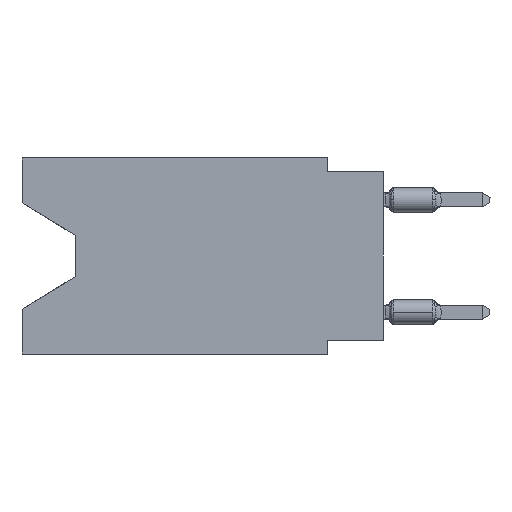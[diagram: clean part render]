
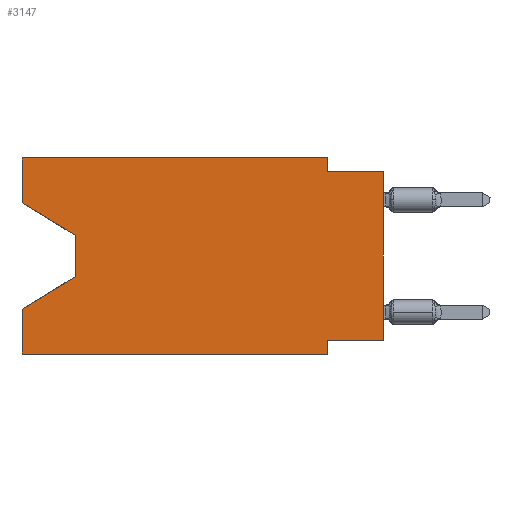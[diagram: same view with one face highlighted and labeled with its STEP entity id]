
A CAD part, left-side view. The second image highlights one B-rep face of the part: STEP entity #3147.
In plain terms, the highlighted planar face has unit normal (-1, 0, 0).
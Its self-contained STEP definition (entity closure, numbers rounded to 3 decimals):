
#388 = EDGE_CURVE ( 'NONE', #33788, #4789, #6880, .T. ) ;
#556 = LINE ( 'NONE', #11380, #32967 ) ;
#1102 = VERTEX_POINT ( 'NONE', #30355 ) ;
#1315 = CARTESIAN_POINT ( 'NONE',  ( 0., 16.383, -8.89 ) ) ;
#1552 = CARTESIAN_POINT ( 'NONE',  ( 0., 16.383, 0. ) ) ;
#1787 = CARTESIAN_POINT ( 'NONE',  ( 0., 0., -8.255 ) ) ;
#2194 = CARTESIAN_POINT ( 'NONE',  ( 0., 16.383, -6.852 ) ) ;
#2644 = VERTEX_POINT ( 'NONE', #27461 ) ;
#3091 = LINE ( 'NONE', #11064, #3766 ) ;
#3147 = ADVANCED_FACE ( 'NONE', ( #27585 ), #18928, .F. ) ;
#3168 = EDGE_CURVE ( 'NONE', #2644, #5817, #12613, .T. ) ;
#3664 = DIRECTION ( 'NONE',  ( 0., 0., -1. ) ) ;
#3766 = VECTOR ( 'NONE', #27421, 1000. ) ;
#4789 = VERTEX_POINT ( 'NONE', #25875 ) ;
#4899 = DIRECTION ( 'NONE',  ( 0., 0., 1. ) ) ;
#5340 = ORIENTED_EDGE ( 'NONE', *, *, #31340, .F. ) ;
#5543 = EDGE_CURVE ( 'NONE', #34579, #11997, #10096, .T. ) ;
#5817 = VERTEX_POINT ( 'NONE', #25352 ) ;
#6232 = VECTOR ( 'NONE', #12568, 1000. ) ;
#6847 = CARTESIAN_POINT ( 'NONE',  ( 0., 13.97, -3.505 ) ) ;
#6880 = LINE ( 'NONE', #1552, #6232 ) ;
#7727 = LINE ( 'NONE', #29780, #26782 ) ;
#8741 = DIRECTION ( 'NONE',  ( 0., 1., 0. ) ) ;
#8787 = CARTESIAN_POINT ( 'NONE',  ( 0., 16.383, 0. ) ) ;
#9070 = VERTEX_POINT ( 'NONE', #15032 ) ;
#9883 = DIRECTION ( 'NONE',  ( 0., -0.855, -0.519 ) ) ;
#10096 = LINE ( 'NONE', #15995, #27792 ) ;
#10443 = EDGE_CURVE ( 'NONE', #27544, #33788, #29067, .T. ) ;
#10603 = ORIENTED_EDGE ( 'NONE', *, *, #388, .F. ) ;
#10645 = CARTESIAN_POINT ( 'NONE',  ( 0., 2.54, -8.89 ) ) ;
#10707 = ORIENTED_EDGE ( 'NONE', *, *, #33769, .T. ) ;
#11064 = CARTESIAN_POINT ( 'NONE',  ( 0., 2.54, 0. ) ) ;
#11380 = CARTESIAN_POINT ( 'NONE',  ( 0., 0., -0.635 ) ) ;
#11549 = DIRECTION ( 'NONE',  ( 0., -1., 0. ) ) ;
#11997 = VERTEX_POINT ( 'NONE', #2194 ) ;
#12079 = AXIS2_PLACEMENT_3D ( 'NONE', #32952, #13908, #21577 ) ;
#12568 = DIRECTION ( 'NONE',  ( 0., -1., 0. ) ) ;
#12613 = LINE ( 'NONE', #1787, #19463 ) ;
#13866 = ORIENTED_EDGE ( 'NONE', *, *, #27496, .T. ) ;
#13908 = DIRECTION ( 'NONE',  ( 1., 0., 0. ) ) ;
#14046 = VECTOR ( 'NONE', #3664, 1000. ) ;
#14711 = ORIENTED_EDGE ( 'NONE', *, *, #5543, .F. ) ;
#15032 = CARTESIAN_POINT ( 'NONE',  ( 0., 2.54, -0.635 ) ) ;
#15124 = CARTESIAN_POINT ( 'NONE',  ( 0., 2.54, -8.89 ) ) ;
#15523 = ORIENTED_EDGE ( 'NONE', *, *, #22405, .T. ) ;
#15639 = LINE ( 'NONE', #10645, #22576 ) ;
#15821 = DIRECTION ( 'NONE',  ( 0., 0., -1. ) ) ;
#15981 = CARTESIAN_POINT ( 'NONE',  ( 0., 13.97, -5.385 ) ) ;
#15995 = CARTESIAN_POINT ( 'NONE',  ( 0., 16.383, 0. ) ) ;
#16669 = LINE ( 'NONE', #15981, #30411 ) ;
#17548 = LINE ( 'NONE', #26055, #21049 ) ;
#18928 = PLANE ( 'NONE',  #12079 ) ;
#19033 = EDGE_CURVE ( 'NONE', #24643, #11997, #16669, .T. ) ;
#19463 = VECTOR ( 'NONE', #8741, 1000. ) ;
#20163 = VECTOR ( 'NONE', #4899, 1000. ) ;
#20191 = ORIENTED_EDGE ( 'NONE', *, *, #19033, .T. ) ;
#20784 = VERTEX_POINT ( 'NONE', #23544 ) ;
#20808 = EDGE_LOOP ( 'NONE', ( #33830, #10707, #20191, #14711, #15523, #32832, #26595, #13866, #5340, #33045, #10603, #28307 ) ) ;
#21049 = VECTOR ( 'NONE', #9883, 1000. ) ;
#21577 = DIRECTION ( 'NONE',  ( 0., 0., -1. ) ) ;
#22405 = EDGE_CURVE ( 'NONE', #34579, #28037, #22628, .T. ) ;
#22576 = VECTOR ( 'NONE', #15821, 1000. ) ;
#22628 = LINE ( 'NONE', #1315, #34583 ) ;
#23544 = CARTESIAN_POINT ( 'NONE',  ( 0., 0., -0.635 ) ) ;
#24643 = VERTEX_POINT ( 'NONE', #29940 ) ;
#25352 = CARTESIAN_POINT ( 'NONE',  ( 0., 2.54, -8.255 ) ) ;
#25875 = CARTESIAN_POINT ( 'NONE',  ( 0., 2.54, 0. ) ) ;
#26055 = CARTESIAN_POINT ( 'NONE',  ( 0., 16.383, -2.038 ) ) ;
#26188 = EDGE_CURVE ( 'NONE', #27544, #1102, #17548, .T. ) ;
#26579 = DIRECTION ( 'NONE',  ( 0., 0., 1. ) ) ;
#26595 = ORIENTED_EDGE ( 'NONE', *, *, #3168, .F. ) ;
#26782 = VECTOR ( 'NONE', #26579, 1000. ) ;
#27421 = DIRECTION ( 'NONE',  ( 0., 0., -1. ) ) ;
#27451 = CARTESIAN_POINT ( 'NONE',  ( 0., 16.383, -2.038 ) ) ;
#27461 = CARTESIAN_POINT ( 'NONE',  ( 0., 0., -8.255 ) ) ;
#27496 = EDGE_CURVE ( 'NONE', #2644, #20784, #7727, .T. ) ;
#27544 = VERTEX_POINT ( 'NONE', #27451 ) ;
#27585 = FACE_OUTER_BOUND ( 'NONE', #20808, .T. ) ;
#27792 = VECTOR ( 'NONE', #34494, 1000. ) ;
#28037 = VERTEX_POINT ( 'NONE', #15124 ) ;
#28307 = ORIENTED_EDGE ( 'NONE', *, *, #10443, .F. ) ;
#29067 = LINE ( 'NONE', #32271, #20163 ) ;
#29460 = DIRECTION ( 'NONE',  ( 0., 0.855, -0.519 ) ) ;
#29780 = CARTESIAN_POINT ( 'NONE',  ( 0., 0., 0. ) ) ;
#29940 = CARTESIAN_POINT ( 'NONE',  ( 0., 13.97, -5.385 ) ) ;
#30355 = CARTESIAN_POINT ( 'NONE',  ( 0., 13.97, -3.505 ) ) ;
#30411 = VECTOR ( 'NONE', #29460, 1000. ) ;
#30452 = DIRECTION ( 'NONE',  ( 0., -1., 0. ) ) ;
#31340 = EDGE_CURVE ( 'NONE', #9070, #20784, #556, .T. ) ;
#32271 = CARTESIAN_POINT ( 'NONE',  ( 0., 16.383, 0. ) ) ;
#32418 = EDGE_CURVE ( 'NONE', #4789, #9070, #3091, .T. ) ;
#32832 = ORIENTED_EDGE ( 'NONE', *, *, #34316, .F. ) ;
#32952 = CARTESIAN_POINT ( 'NONE',  ( 0., 16.383, 0. ) ) ;
#32967 = VECTOR ( 'NONE', #11549, 1000. ) ;
#33045 = ORIENTED_EDGE ( 'NONE', *, *, #32418, .F. ) ;
#33166 = LINE ( 'NONE', #6847, #14046 ) ;
#33769 = EDGE_CURVE ( 'NONE', #1102, #24643, #33166, .T. ) ;
#33788 = VERTEX_POINT ( 'NONE', #8787 ) ;
#33830 = ORIENTED_EDGE ( 'NONE', *, *, #26188, .T. ) ;
#34316 = EDGE_CURVE ( 'NONE', #5817, #28037, #15639, .T. ) ;
#34494 = DIRECTION ( 'NONE',  ( 0., 0., 1. ) ) ;
#34579 = VERTEX_POINT ( 'NONE', #34997 ) ;
#34583 = VECTOR ( 'NONE', #30452, 1000. ) ;
#34997 = CARTESIAN_POINT ( 'NONE',  ( 0., 16.383, -8.89 ) ) ;
